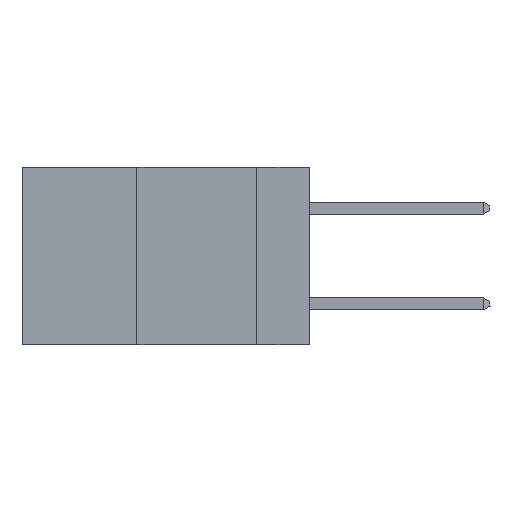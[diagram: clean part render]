
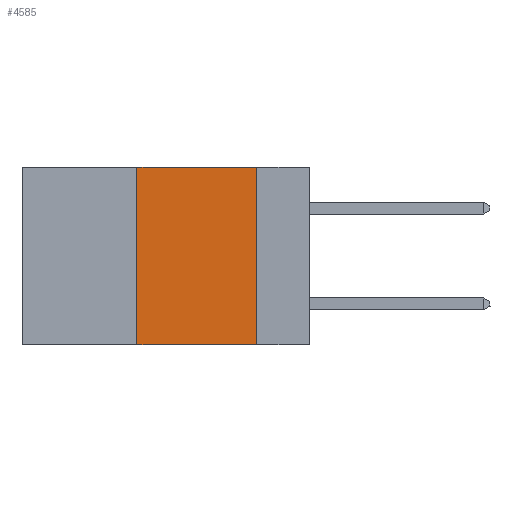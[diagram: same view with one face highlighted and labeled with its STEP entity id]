
A CAD part, left-side view. The second image highlights one B-rep face of the part: STEP entity #4585.
In plain terms, the highlighted planar face has unit normal (-1, 0, 0).
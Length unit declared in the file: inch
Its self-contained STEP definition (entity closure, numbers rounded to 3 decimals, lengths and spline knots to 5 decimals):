
#1874 = CARTESIAN_POINT ( 'NONE',  ( 0., 0.6, -0.37 ) ) ;
#2304 = ORIENTED_EDGE ( 'NONE', *, *, #24330, .F. ) ;
#2789 = VECTOR ( 'NONE', #8466, 39.37008 ) ;
#3334 = CARTESIAN_POINT ( 'NONE',  ( 0., 0.6, 0. ) ) ;
#3432 = FACE_OUTER_BOUND ( 'NONE', #7980, .T. ) ;
#4151 = EDGE_CURVE ( 'NONE', #17279, #5512, #15956, .T. ) ;
#4177 = VERTEX_POINT ( 'NONE', #25744 ) ;
#4585 = ADVANCED_FACE ( 'NONE', ( #3432 ), #20494, .F. ) ;
#5512 = VERTEX_POINT ( 'NONE', #5938 ) ;
#5522 = DIRECTION ( 'NONE',  ( 0., 0., -1. ) ) ;
#5669 = DIRECTION ( 'NONE',  ( 0., 0., -1. ) ) ;
#5938 = CARTESIAN_POINT ( 'NONE',  ( 0., 0.36, 0. ) ) ;
#7653 = CARTESIAN_POINT ( 'NONE',  ( 0., 0.11, 0. ) ) ;
#7980 = EDGE_LOOP ( 'NONE', ( #15718, #2304, #10753, #14550 ) ) ;
#8466 = DIRECTION ( 'NONE',  ( 0., 0., 1. ) ) ;
#8653 = CARTESIAN_POINT ( 'NONE',  ( 0., 0.36, 0. ) ) ;
#8667 = VERTEX_POINT ( 'NONE', #14472 ) ;
#8729 = VECTOR ( 'NONE', #23088, 39.37008 ) ;
#9296 = LINE ( 'NONE', #7653, #18091 ) ;
#10753 = ORIENTED_EDGE ( 'NONE', *, *, #4151, .F. ) ;
#13532 = LINE ( 'NONE', #1874, #20925 ) ;
#14472 = CARTESIAN_POINT ( 'NONE',  ( 0., 0.11, 0. ) ) ;
#14550 = ORIENTED_EDGE ( 'NONE', *, *, #22537, .T. ) ;
#15718 = ORIENTED_EDGE ( 'NONE', *, *, #19976, .F. ) ;
#15956 = LINE ( 'NONE', #8653, #2789 ) ;
#16386 = CARTESIAN_POINT ( 'NONE',  ( 0., 0.6, 0. ) ) ;
#16995 = DIRECTION ( 'NONE',  ( 0., -1., 0. ) ) ;
#17279 = VERTEX_POINT ( 'NONE', #20763 ) ;
#18091 = VECTOR ( 'NONE', #5669, 39.37008 ) ;
#19976 = EDGE_CURVE ( 'NONE', #8667, #4177, #9296, .T. ) ;
#20494 = PLANE ( 'NONE',  #21043 ) ;
#20504 = LINE ( 'NONE', #16386, #8729 ) ;
#20763 = CARTESIAN_POINT ( 'NONE',  ( 0., 0.36, -0.37 ) ) ;
#20925 = VECTOR ( 'NONE', #16995, 39.37008 ) ;
#21043 = AXIS2_PLACEMENT_3D ( 'NONE', #3334, #27362, #5522 ) ;
#22537 = EDGE_CURVE ( 'NONE', #17279, #4177, #13532, .T. ) ;
#23088 = DIRECTION ( 'NONE',  ( 0., -1., 0. ) ) ;
#24330 = EDGE_CURVE ( 'NONE', #5512, #8667, #20504, .T. ) ;
#25744 = CARTESIAN_POINT ( 'NONE',  ( 0., 0.11, -0.37 ) ) ;
#27362 = DIRECTION ( 'NONE',  ( 1., 0., 0. ) ) ;
